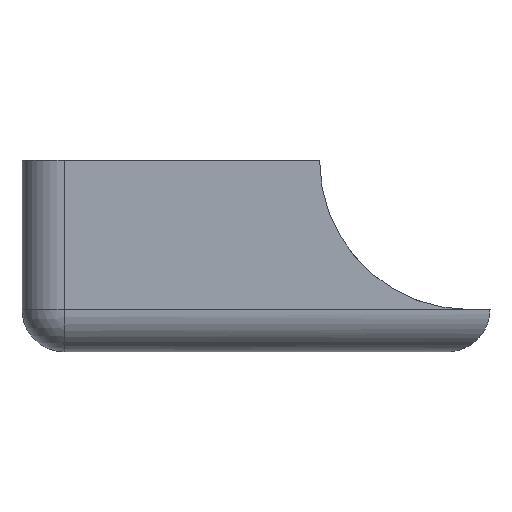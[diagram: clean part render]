
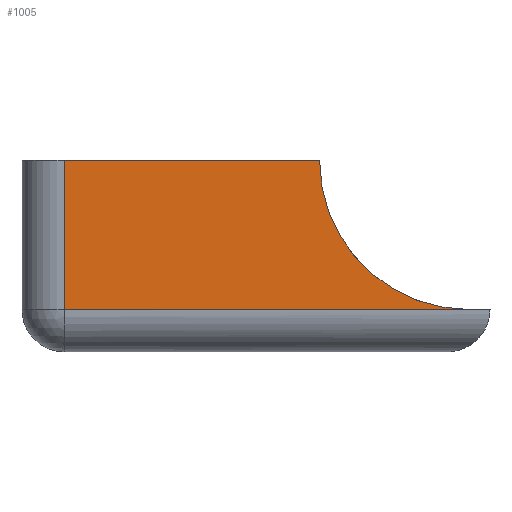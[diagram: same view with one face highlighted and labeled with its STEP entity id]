
A CAD part, left-side view. The second image highlights one B-rep face of the part: STEP entity #1005.
In plain terms, the highlighted planar face has unit normal (-1, 0, 0).
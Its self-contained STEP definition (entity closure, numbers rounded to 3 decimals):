
#8 = CARTESIAN_POINT ( 'NONE',  ( -29.771, 18.468, 107.492 ) ) ;
#38 = VERTEX_POINT ( 'NONE', #851 ) ;
#46 = VERTEX_POINT ( 'NONE', #1102 ) ;
#125 = DIRECTION ( 'NONE',  ( 0., 0., -1. ) ) ;
#154 = LINE ( 'NONE', #613, #790 ) ;
#209 = CARTESIAN_POINT ( 'NONE',  ( -29.771, 18.468, 76.289 ) ) ;
#363 = AXIS2_PLACEMENT_3D ( 'NONE', #8, #876, #125 ) ;
#416 = AXIS2_PLACEMENT_3D ( 'NONE', #496, #1374, #629 ) ;
#418 = ORIENTED_EDGE ( 'NONE', *, *, #906, .F. ) ;
#424 = ORIENTED_EDGE ( 'NONE', *, *, #1306, .F. ) ;
#496 = CARTESIAN_POINT ( 'NONE',  ( -29.771, 19.468, 76.289 ) ) ;
#552 = EDGE_CURVE ( 'NONE', #46, #905, #725, .T. ) ;
#588 = ORIENTED_EDGE ( 'NONE', *, *, #1550, .T. ) ;
#613 = CARTESIAN_POINT ( 'NONE',  ( -29.771, 18.468, 69.232 ) ) ;
#619 = ORIENTED_EDGE ( 'NONE', *, *, #552, .T. ) ;
#629 = DIRECTION ( 'NONE',  ( 0., 0., -1. ) ) ;
#696 = EDGE_LOOP ( 'NONE', ( #619, #588, #424, #418 ) ) ;
#725 = LINE ( 'NONE', #1272, #768 ) ;
#768 = VECTOR ( 'NONE', #1402, 1000. ) ;
#790 = VECTOR ( 'NONE', #865, 1000. ) ;
#851 = CARTESIAN_POINT ( 'NONE',  ( -29.771, 19.468, 69.232 ) ) ;
#852 = FACE_OUTER_BOUND ( 'NONE', #696, .T. ) ;
#865 = DIRECTION ( 'NONE',  ( 0., -1., 0. ) ) ;
#876 = DIRECTION ( 'NONE',  ( -1., 0., 0. ) ) ;
#905 = VERTEX_POINT ( 'NONE', #1085 ) ;
#906 = EDGE_CURVE ( 'NONE', #46, #1144, #968, .T. ) ;
#924 = VECTOR ( 'NONE', #1591, 1000. ) ;
#968 = LINE ( 'NONE', #209, #924 ) ;
#972 = PLANE ( 'NONE',  #363 ) ;
#1005 = ADVANCED_FACE ( 'NONE', ( #852 ), #972, .T. ) ;
#1059 = CARTESIAN_POINT ( 'NONE',  ( -29.771, 26.525, 76.289 ) ) ;
#1085 = CARTESIAN_POINT ( 'NONE',  ( -29.771, 38.59, 69.232 ) ) ;
#1102 = CARTESIAN_POINT ( 'NONE',  ( -29.771, 38.59, 76.289 ) ) ;
#1144 = VERTEX_POINT ( 'NONE', #1059 ) ;
#1272 = CARTESIAN_POINT ( 'NONE',  ( -29.771, 38.59, 107.492 ) ) ;
#1306 = EDGE_CURVE ( 'NONE', #1144, #38, #1322, .T. ) ;
#1322 = CIRCLE ( 'NONE', #416, 7.057 ) ;
#1374 = DIRECTION ( 'NONE',  ( -1., 0., 0. ) ) ;
#1402 = DIRECTION ( 'NONE',  ( 0., 0., -1. ) ) ;
#1550 = EDGE_CURVE ( 'NONE', #905, #38, #154, .T. ) ;
#1591 = DIRECTION ( 'NONE',  ( 0., -1., 0. ) ) ;
